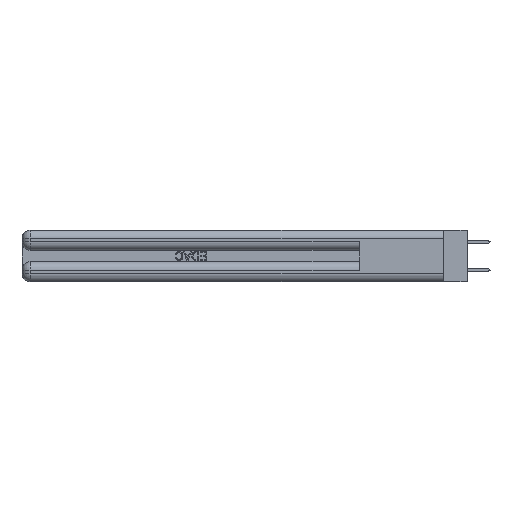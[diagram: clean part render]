
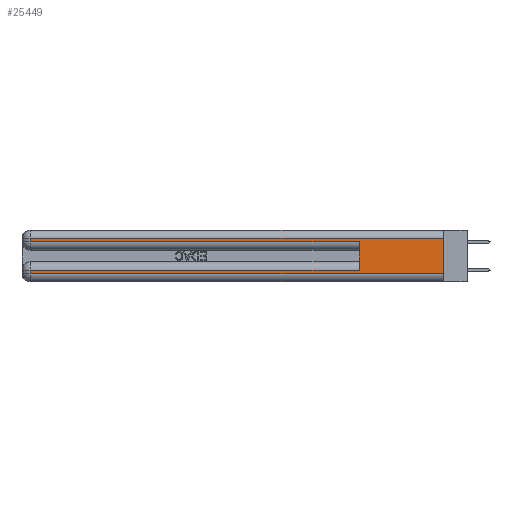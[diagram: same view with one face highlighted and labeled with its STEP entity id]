
A CAD part, left-side view. The second image highlights one B-rep face of the part: STEP entity #25449.
In plain terms, the highlighted planar face has unit normal (-1, 0, 0).
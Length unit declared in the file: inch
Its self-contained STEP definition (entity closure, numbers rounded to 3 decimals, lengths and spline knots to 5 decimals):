
#672 = ORIENTED_EDGE ( 'NONE', *, *, #15557, .F. ) ;
#769 = CARTESIAN_POINT ( 'NONE',  ( 0., 0.6, 0.085 ) ) ;
#1589 = LINE ( 'NONE', #35455, #11822 ) ;
#1721 = VERTEX_POINT ( 'NONE', #23462 ) ;
#1870 = ORIENTED_EDGE ( 'NONE', *, *, #20706, .T. ) ;
#1988 = LINE ( 'NONE', #16033, #32574 ) ;
#2279 = ORIENTED_EDGE ( 'NONE', *, *, #28575, .T. ) ;
#2321 = CARTESIAN_POINT ( 'NONE',  ( 0., 2.94, 0.31 ) ) ;
#2629 = LINE ( 'NONE', #5683, #9566 ) ;
#4378 = AXIS2_PLACEMENT_3D ( 'NONE', #25141, #34078, #4411 ) ;
#4411 = DIRECTION ( 'NONE',  ( 0., 0., -1. ) ) ;
#4422 = DIRECTION ( 'NONE',  ( 0., 0., -1. ) ) ;
#4784 = PLANE ( 'NONE',  #4378 ) ;
#5067 = VERTEX_POINT ( 'NONE', #2321 ) ;
#5600 = ORIENTED_EDGE ( 'NONE', *, *, #23393, .T. ) ;
#5683 = CARTESIAN_POINT ( 'NONE',  ( 0., 0., 0.085 ) ) ;
#6572 = DIRECTION ( 'NONE',  ( 0., 0., -1. ) ) ;
#7688 = LINE ( 'NONE', #8930, #32247 ) ;
#7705 = VERTEX_POINT ( 'NONE', #33900 ) ;
#7850 = CARTESIAN_POINT ( 'NONE',  ( 0., 0., 0.285 ) ) ;
#8655 = VECTOR ( 'NONE', #22201, 39.37008 ) ;
#8930 = CARTESIAN_POINT ( 'NONE',  ( 0., 2.94, 0.37 ) ) ;
#9445 = CARTESIAN_POINT ( 'NONE',  ( 0., 2.94, 0.085 ) ) ;
#9566 = VECTOR ( 'NONE', #24687, 39.37008 ) ;
#9894 = EDGE_CURVE ( 'NONE', #14026, #9993, #1988, .T. ) ;
#9993 = VERTEX_POINT ( 'NONE', #19309 ) ;
#10356 = VECTOR ( 'NONE', #10436, 39.37008 ) ;
#10436 = DIRECTION ( 'NONE',  ( 0., -1., 0. ) ) ;
#10527 = CARTESIAN_POINT ( 'NONE',  ( 0., 0., 0.06 ) ) ;
#10957 = CARTESIAN_POINT ( 'NONE',  ( 0., 0., 0.06 ) ) ;
#11447 = VECTOR ( 'NONE', #18707, 39.37008 ) ;
#11822 = VECTOR ( 'NONE', #20211, 39.37008 ) ;
#13591 = LINE ( 'NONE', #7850, #10356 ) ;
#14026 = VERTEX_POINT ( 'NONE', #769 ) ;
#14583 = ORIENTED_EDGE ( 'NONE', *, *, #9894, .F. ) ;
#15557 = EDGE_CURVE ( 'NONE', #29037, #27228, #19335, .T. ) ;
#16033 = CARTESIAN_POINT ( 'NONE',  ( 0., 0.6, 0.145 ) ) ;
#16150 = ORIENTED_EDGE ( 'NONE', *, *, #34584, .T. ) ;
#16499 = LINE ( 'NONE', #27092, #29451 ) ;
#18707 = DIRECTION ( 'NONE',  ( 0., 0., -1. ) ) ;
#19309 = CARTESIAN_POINT ( 'NONE',  ( 0., 0.6, 0.285 ) ) ;
#19335 = LINE ( 'NONE', #27841, #11447 ) ;
#20131 = EDGE_CURVE ( 'NONE', #14026, #23595, #2629, .T. ) ;
#20211 = DIRECTION ( 'NONE',  ( 0., 1., 0. ) ) ;
#20604 = EDGE_CURVE ( 'NONE', #5067, #1721, #7688, .T. ) ;
#20706 = EDGE_CURVE ( 'NONE', #23595, #7705, #16499, .T. ) ;
#22201 = DIRECTION ( 'NONE',  ( 0., -1., 0. ) ) ;
#22740 = CARTESIAN_POINT ( 'NONE',  ( 0., 0., 0.31 ) ) ;
#23393 = EDGE_CURVE ( 'NONE', #1721, #9993, #13591, .T. ) ;
#23462 = CARTESIAN_POINT ( 'NONE',  ( 0., 2.94, 0.285 ) ) ;
#23595 = VERTEX_POINT ( 'NONE', #9445 ) ;
#24687 = DIRECTION ( 'NONE',  ( 0., 1., 0. ) ) ;
#25141 = CARTESIAN_POINT ( 'NONE',  ( 0., 0., 0.37 ) ) ;
#25449 = ADVANCED_FACE ( 'NONE', ( #37546 ), #4784, .F. ) ;
#27092 = CARTESIAN_POINT ( 'NONE',  ( 0., 2.94, 0.37 ) ) ;
#27228 = VERTEX_POINT ( 'NONE', #10957 ) ;
#27841 = CARTESIAN_POINT ( 'NONE',  ( 0., 0., 0.37 ) ) ;
#28575 = EDGE_CURVE ( 'NONE', #29037, #5067, #1589, .T. ) ;
#28948 = ORIENTED_EDGE ( 'NONE', *, *, #20131, .T. ) ;
#29037 = VERTEX_POINT ( 'NONE', #22740 ) ;
#29451 = VECTOR ( 'NONE', #4422, 39.37008 ) ;
#29581 = EDGE_LOOP ( 'NONE', ( #672, #2279, #35482, #5600, #14583, #28948, #1870, #16150 ) ) ;
#32247 = VECTOR ( 'NONE', #6572, 39.37008 ) ;
#32574 = VECTOR ( 'NONE', #36764, 39.37008 ) ;
#33900 = CARTESIAN_POINT ( 'NONE',  ( 0., 2.94, 0.06 ) ) ;
#34078 = DIRECTION ( 'NONE',  ( 1., 0., 0. ) ) ;
#34584 = EDGE_CURVE ( 'NONE', #7705, #27228, #37858, .T. ) ;
#35455 = CARTESIAN_POINT ( 'NONE',  ( 0., 0., 0.31 ) ) ;
#35482 = ORIENTED_EDGE ( 'NONE', *, *, #20604, .T. ) ;
#36764 = DIRECTION ( 'NONE',  ( 0., 0., 1. ) ) ;
#37546 = FACE_OUTER_BOUND ( 'NONE', #29581, .T. ) ;
#37858 = LINE ( 'NONE', #10527, #8655 ) ;
